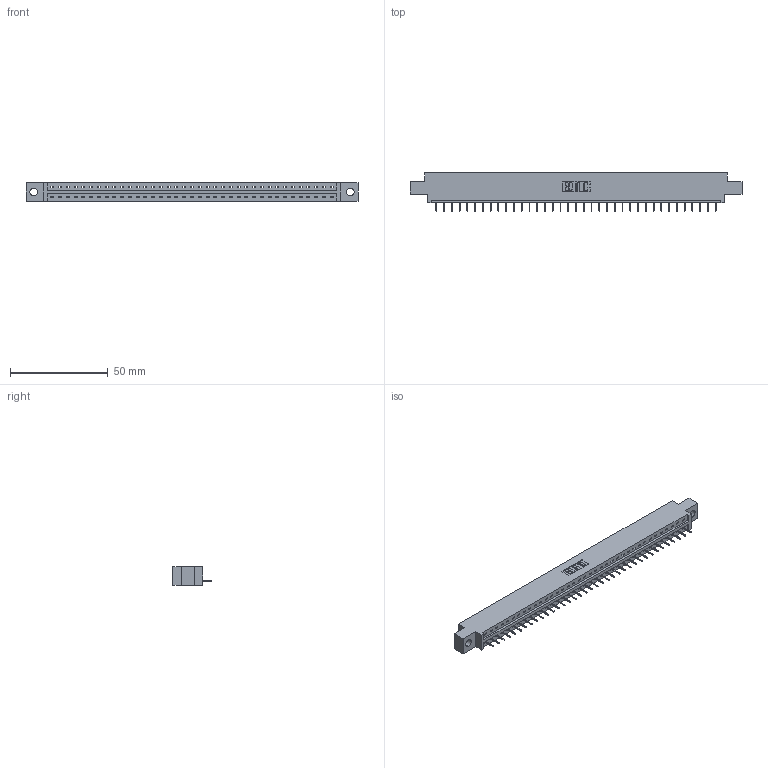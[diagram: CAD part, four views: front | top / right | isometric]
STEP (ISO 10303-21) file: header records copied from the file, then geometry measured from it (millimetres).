
FILE_DESCRIPTION (( 'STEP AP203' ), '1' );
FILE_NAME ('337-037-524-604.STEP', '2019-10-01T15:27:55', ( '' ), ( '' ), 'SwSTEP 2.0', 'SolidWorks 2016', '' );
FILE_SCHEMA (( 'CONFIG_CONTROL_DESIGN' ));
Length unit declared in the file: inch
Products named in the file (3): 337 Part_0.170 Offset - 0.156 Dia-TH; 337-037-524-604; 345-292-001_345-293-124
Assembly tree (38 placements, depth 2):
  337-037-524-604
    337 Part_0.170 Offset - 0.156 Dia-TH
    345-292-001_345-293-124  x37
Bounding box: 169.62 x 19.69 x 9.4 mm (x, y, z)
Volume: 17215.2 mm3; surface area: 17139.3 mm2
Topology: 38 solids, 38 shells, 2560 faces, 7427 edges, 4802 vertices
Faces by surface type: plane 1998, cylinder 562
Entity records: 28359 total; most frequent: CARTESIAN_POINT 4945, ORIENTED_EDGE 4918, DIRECTION 4173, EDGE_CURVE 2459, VECTOR 2335, LINE 2335, VERTEX_POINT 1634, AXIS2_PLACEMENT_3D 919
